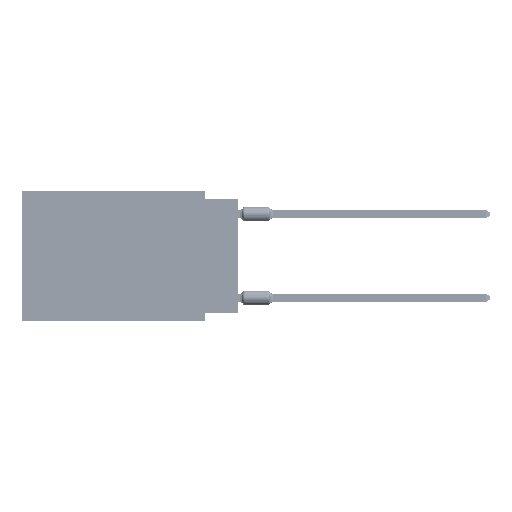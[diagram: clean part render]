
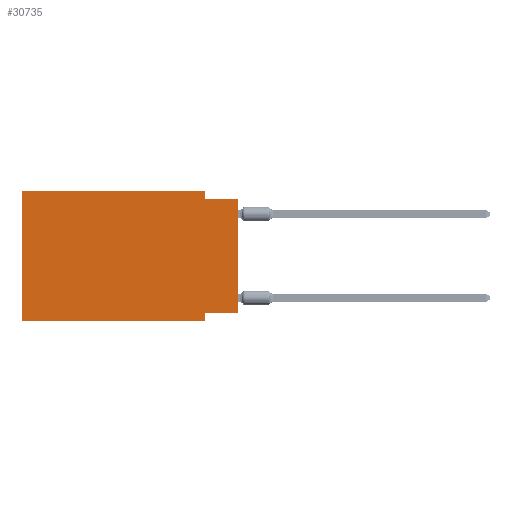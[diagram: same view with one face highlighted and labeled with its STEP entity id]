
A CAD part, left-side view. The second image highlights one B-rep face of the part: STEP entity #30735.
In plain terms, the highlighted planar face has unit normal (-1, 0, 0).
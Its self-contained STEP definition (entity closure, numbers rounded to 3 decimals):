
#230 = ORIENTED_EDGE ( 'NONE', *, *, #37748, .F. ) ;
#2032 = ORIENTED_EDGE ( 'NONE', *, *, #18161, .F. ) ;
#2640 = DIRECTION ( 'NONE',  ( 0., -1., 0. ) ) ;
#2984 = VERTEX_POINT ( 'NONE', #4070 ) ;
#3006 = LINE ( 'NONE', #54355, #26451 ) ;
#3844 = VERTEX_POINT ( 'NONE', #4167 ) ;
#4070 = CARTESIAN_POINT ( 'NONE',  ( 0., 0., -0.635 ) ) ;
#4167 = CARTESIAN_POINT ( 'NONE',  ( 0., 2.54, -0.635 ) ) ;
#6655 = EDGE_CURVE ( 'NONE', #50575, #29320, #3006, .T. ) ;
#7398 = ORIENTED_EDGE ( 'NONE', *, *, #6655, .T. ) ;
#8705 = CARTESIAN_POINT ( 'NONE',  ( 0., 2.54, 0. ) ) ;
#10157 = DIRECTION ( 'NONE',  ( 0., -1., 0. ) ) ;
#10895 = LINE ( 'NONE', #28591, #35178 ) ;
#15412 = VERTEX_POINT ( 'NONE', #74257 ) ;
#15631 = DIRECTION ( 'NONE',  ( 0., 0., 1. ) ) ;
#17902 = ORIENTED_EDGE ( 'NONE', *, *, #26667, .F. ) ;
#18093 = VERTEX_POINT ( 'NONE', #25573 ) ;
#18161 = EDGE_CURVE ( 'NONE', #50575, #18093, #62701, .T. ) ;
#21275 = LINE ( 'NONE', #67338, #54743 ) ;
#21825 = EDGE_CURVE ( 'NONE', #18093, #31731, #56805, .T. ) ;
#22322 = DIRECTION ( 'NONE',  ( 0., 0., 1. ) ) ;
#22352 = VECTOR ( 'NONE', #22322, 1000. ) ;
#25573 = CARTESIAN_POINT ( 'NONE',  ( 0., 16.383, 0. ) ) ;
#26451 = VECTOR ( 'NONE', #2640, 1000. ) ;
#26667 = EDGE_CURVE ( 'NONE', #63304, #29320, #66133, .T. ) ;
#27333 = CARTESIAN_POINT ( 'NONE',  ( 0., 2.54, -9.906 ) ) ;
#27906 = AXIS2_PLACEMENT_3D ( 'NONE', #47404, #52680, #37172 ) ;
#28591 = CARTESIAN_POINT ( 'NONE',  ( 0., 0., -0.635 ) ) ;
#28595 = EDGE_LOOP ( 'NONE', ( #36069, #29817, #63142, #70633, #2032, #7398, #17902, #230 ) ) ;
#29320 = VERTEX_POINT ( 'NONE', #27333 ) ;
#29471 = CARTESIAN_POINT ( 'NONE',  ( 0., 2.54, -9.271 ) ) ;
#29817 = ORIENTED_EDGE ( 'NONE', *, *, #40882, .F. ) ;
#30216 = VECTOR ( 'NONE', #43744, 1000. ) ;
#30735 = ADVANCED_FACE ( 'NONE', ( #65524 ), #35678, .F. ) ;
#31731 = VERTEX_POINT ( 'NONE', #40993 ) ;
#32651 = DIRECTION ( 'NONE',  ( 0., -1., 0. ) ) ;
#32883 = DIRECTION ( 'NONE',  ( 0., 0., -1. ) ) ;
#34686 = VECTOR ( 'NONE', #42290, 1000. ) ;
#35178 = VECTOR ( 'NONE', #10157, 1000. ) ;
#35678 = PLANE ( 'NONE',  #27906 ) ;
#36069 = ORIENTED_EDGE ( 'NONE', *, *, #65305, .T. ) ;
#36946 = LINE ( 'NONE', #43356, #30216 ) ;
#37172 = DIRECTION ( 'NONE',  ( 0., 0., -1. ) ) ;
#37748 = EDGE_CURVE ( 'NONE', #15412, #63304, #36946, .T. ) ;
#40882 = EDGE_CURVE ( 'NONE', #3844, #2984, #10895, .T. ) ;
#40993 = CARTESIAN_POINT ( 'NONE',  ( 0., 2.54, 0. ) ) ;
#42290 = DIRECTION ( 'NONE',  ( 0., 0., -1. ) ) ;
#43356 = CARTESIAN_POINT ( 'NONE',  ( 0., 0., -9.271 ) ) ;
#43744 = DIRECTION ( 'NONE',  ( 0., 1., 0. ) ) ;
#47030 = VECTOR ( 'NONE', #32883, 1000. ) ;
#47404 = CARTESIAN_POINT ( 'NONE',  ( 0., 16.383, 0. ) ) ;
#50575 = VERTEX_POINT ( 'NONE', #62695 ) ;
#52680 = DIRECTION ( 'NONE',  ( 1., 0., 0. ) ) ;
#53246 = EDGE_CURVE ( 'NONE', #31731, #3844, #60774, .T. ) ;
#54355 = CARTESIAN_POINT ( 'NONE',  ( 0., 16.383, -9.906 ) ) ;
#54743 = VECTOR ( 'NONE', #15631, 1000. ) ;
#55924 = CARTESIAN_POINT ( 'NONE',  ( 0., 2.54, -9.906 ) ) ;
#56360 = VECTOR ( 'NONE', #32651, 1000. ) ;
#56429 = CARTESIAN_POINT ( 'NONE',  ( 0., 16.383, 0. ) ) ;
#56805 = LINE ( 'NONE', #56429, #56360 ) ;
#60774 = LINE ( 'NONE', #8705, #34686 ) ;
#61964 = CARTESIAN_POINT ( 'NONE',  ( 0., 16.383, 0. ) ) ;
#62695 = CARTESIAN_POINT ( 'NONE',  ( 0., 16.383, -9.906 ) ) ;
#62701 = LINE ( 'NONE', #61964, #22352 ) ;
#63142 = ORIENTED_EDGE ( 'NONE', *, *, #53246, .F. ) ;
#63304 = VERTEX_POINT ( 'NONE', #29471 ) ;
#65305 = EDGE_CURVE ( 'NONE', #15412, #2984, #21275, .T. ) ;
#65524 = FACE_OUTER_BOUND ( 'NONE', #28595, .T. ) ;
#66133 = LINE ( 'NONE', #55924, #47030 ) ;
#67338 = CARTESIAN_POINT ( 'NONE',  ( 0., 0., 0. ) ) ;
#70633 = ORIENTED_EDGE ( 'NONE', *, *, #21825, .F. ) ;
#74257 = CARTESIAN_POINT ( 'NONE',  ( 0., 0., -9.271 ) ) ;
